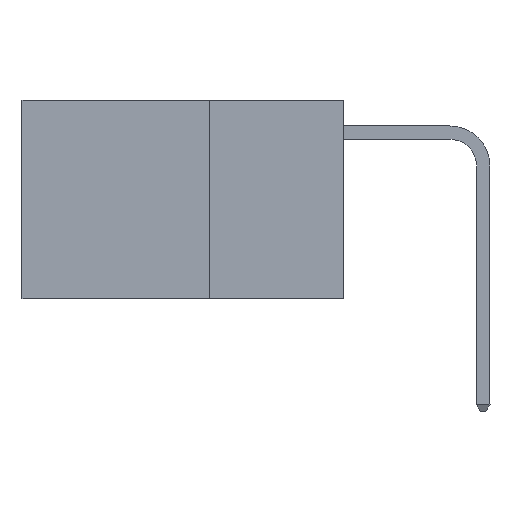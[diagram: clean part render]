
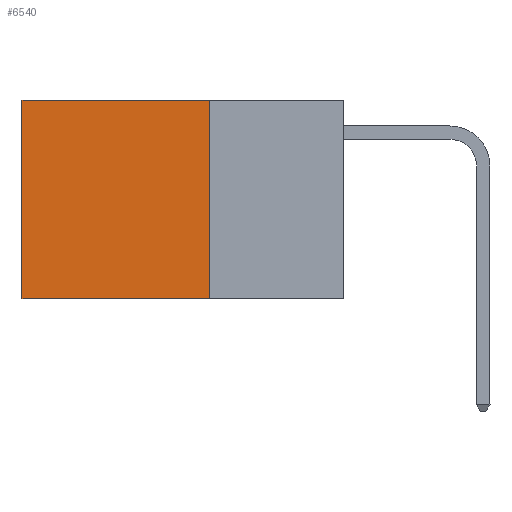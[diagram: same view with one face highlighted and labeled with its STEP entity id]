
A CAD part, left-side view. The second image highlights one B-rep face of the part: STEP entity #6540.
In plain terms, the highlighted planar face has unit normal (-1, 0, 0).
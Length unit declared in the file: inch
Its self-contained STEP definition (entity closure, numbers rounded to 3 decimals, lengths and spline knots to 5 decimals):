
#501 = CARTESIAN_POINT ( 'NONE',  ( 0.2625, 0.25, 0. ) ) ;
#872 = CARTESIAN_POINT ( 'NONE',  ( 0.2625, 0.25, -0.37 ) ) ;
#1140 = VECTOR ( 'NONE', #3874, 39.37008 ) ;
#1276 = CARTESIAN_POINT ( 'NONE',  ( 0.2625, 0.25, 0. ) ) ;
#1348 = PLANE ( 'NONE',  #1478 ) ;
#1478 = AXIS2_PLACEMENT_3D ( 'NONE', #501, #4388, #9795 ) ;
#2402 = ORIENTED_EDGE ( 'NONE', *, *, #6350, .F. ) ;
#2827 = EDGE_CURVE ( 'NONE', #9754, #6757, #3056, .T. ) ;
#3056 = LINE ( 'NONE', #11300, #5326 ) ;
#3165 = LINE ( 'NONE', #7568, #1140 ) ;
#3874 = DIRECTION ( 'NONE',  ( 0., 0., -1. ) ) ;
#3993 = ORIENTED_EDGE ( 'NONE', *, *, #10569, .F. ) ;
#4048 = VECTOR ( 'NONE', #11912, 39.37008 ) ;
#4388 = DIRECTION ( 'NONE',  ( 1., 0., 0. ) ) ;
#5326 = VECTOR ( 'NONE', #6746, 39.37008 ) ;
#6150 = FACE_OUTER_BOUND ( 'NONE', #7797, .T. ) ;
#6326 = VECTOR ( 'NONE', #8694, 39.37008 ) ;
#6350 = EDGE_CURVE ( 'NONE', #9754, #6544, #7894, .T. ) ;
#6540 = ADVANCED_FACE ( 'NONE', ( #6150 ), #1348, .F. ) ;
#6544 = VERTEX_POINT ( 'NONE', #9852 ) ;
#6746 = DIRECTION ( 'NONE',  ( 0., 1., 0. ) ) ;
#6757 = VERTEX_POINT ( 'NONE', #9396 ) ;
#7568 = CARTESIAN_POINT ( 'NONE',  ( 0.2625, 0.6, 0. ) ) ;
#7797 = EDGE_LOOP ( 'NONE', ( #10220, #3993, #2402, #10836 ) ) ;
#7894 = LINE ( 'NONE', #1276, #6326 ) ;
#8102 = LINE ( 'NONE', #872, #4048 ) ;
#8146 = CARTESIAN_POINT ( 'NONE',  ( 0.2625, 0.25, 0. ) ) ;
#8694 = DIRECTION ( 'NONE',  ( 0., 0., -1. ) ) ;
#9396 = CARTESIAN_POINT ( 'NONE',  ( 0.2625, 0.6, 0. ) ) ;
#9754 = VERTEX_POINT ( 'NONE', #8146 ) ;
#9795 = DIRECTION ( 'NONE',  ( 0., 0., -1. ) ) ;
#9852 = CARTESIAN_POINT ( 'NONE',  ( 0.2625, 0.25, -0.37 ) ) ;
#10220 = ORIENTED_EDGE ( 'NONE', *, *, #11150, .T. ) ;
#10547 = VERTEX_POINT ( 'NONE', #10956 ) ;
#10569 = EDGE_CURVE ( 'NONE', #6544, #10547, #8102, .T. ) ;
#10836 = ORIENTED_EDGE ( 'NONE', *, *, #2827, .T. ) ;
#10956 = CARTESIAN_POINT ( 'NONE',  ( 0.2625, 0.6, -0.37 ) ) ;
#11150 = EDGE_CURVE ( 'NONE', #6757, #10547, #3165, .T. ) ;
#11300 = CARTESIAN_POINT ( 'NONE',  ( 0.2625, 0.25, 0. ) ) ;
#11912 = DIRECTION ( 'NONE',  ( 0., 1., 0. ) ) ;
